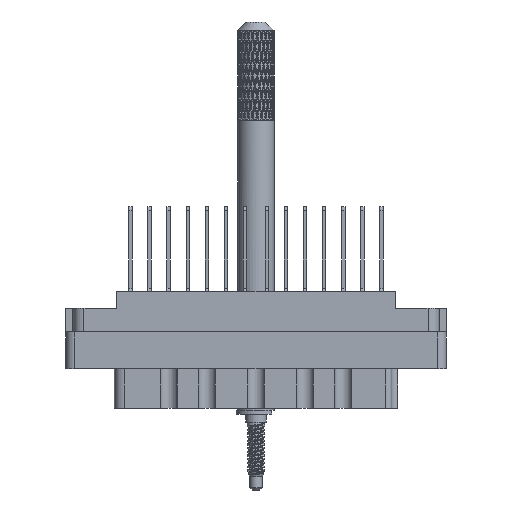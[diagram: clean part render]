
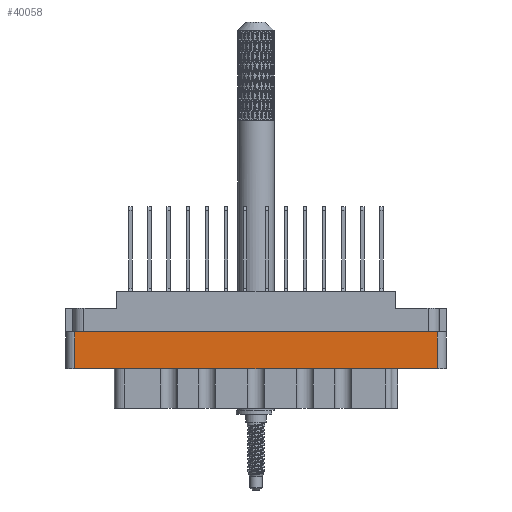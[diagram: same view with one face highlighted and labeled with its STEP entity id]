
A CAD part, front view. The second image highlights one B-rep face of the part: STEP entity #40058.
In plain terms, the highlighted planar face has unit normal (0, -1, 0).
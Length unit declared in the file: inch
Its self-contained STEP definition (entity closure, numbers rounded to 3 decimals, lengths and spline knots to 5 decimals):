
#10242 = DIRECTION ( 'NONE',  ( 0., -1., 0. ) ) ;
#10829 = FACE_OUTER_BOUND ( 'NONE', #108173, .T. ) ;
#15370 = ORIENTED_EDGE ( 'NONE', *, *, #99197, .F. ) ;
#15640 = CARTESIAN_POINT ( 'NONE',  ( 1.234, -0.438, -0.798 ) ) ;
#28020 = CARTESIAN_POINT ( 'NONE',  ( 0., -0.438, -0.529 ) ) ;
#29146 = CARTESIAN_POINT ( 'NONE',  ( -1.296, -0.438, -0.798 ) ) ;
#30642 = VERTEX_POINT ( 'NONE', #67618 ) ;
#34133 = DIRECTION ( 'NONE',  ( 0., 0., 1. ) ) ;
#37574 = VECTOR ( 'NONE', #46187, 39.37008 ) ;
#40058 = ADVANCED_FACE ( 'NONE', ( #10829 ), #91553, .T. ) ;
#45453 = ORIENTED_EDGE ( 'NONE', *, *, #83972, .F. ) ;
#46187 = DIRECTION ( 'NONE',  ( -1., 0., 0. ) ) ;
#47696 = DIRECTION ( 'NONE',  ( 0., 0., -1. ) ) ;
#49964 = AXIS2_PLACEMENT_3D ( 'NONE', #29146, #10242, #47696 ) ;
#51877 = CARTESIAN_POINT ( 'NONE',  ( 1.234, -0.438, -0.277 ) ) ;
#53522 = DIRECTION ( 'NONE',  ( 1., 0., 0. ) ) ;
#61423 = VERTEX_POINT ( 'NONE', #98308 ) ;
#61961 = DIRECTION ( 'NONE',  ( 0., 0., -1. ) ) ;
#67618 = CARTESIAN_POINT ( 'NONE',  ( -1.234, -0.438, -0.529 ) ) ;
#68690 = VERTEX_POINT ( 'NONE', #51877 ) ;
#70128 = CARTESIAN_POINT ( 'NONE',  ( 0., -0.438, -0.277 ) ) ;
#71043 = CARTESIAN_POINT ( 'NONE',  ( -1.234, -0.438, -0.798 ) ) ;
#77001 = VECTOR ( 'NONE', #53522, 39.37008 ) ;
#78864 = VECTOR ( 'NONE', #61961, 39.37008 ) ;
#79878 = LINE ( 'NONE', #70128, #77001 ) ;
#81186 = VERTEX_POINT ( 'NONE', #84804 ) ;
#81673 = LINE ( 'NONE', #71043, #78864 ) ;
#83972 = EDGE_CURVE ( 'NONE', #61423, #68690, #79878, .T. ) ;
#84804 = CARTESIAN_POINT ( 'NONE',  ( 1.234, -0.438, -0.529 ) ) ;
#87998 = VECTOR ( 'NONE', #34133, 39.37008 ) ;
#90091 = ORIENTED_EDGE ( 'NONE', *, *, #114015, .T. ) ;
#91553 = PLANE ( 'NONE',  #49964 ) ;
#91884 = ORIENTED_EDGE ( 'NONE', *, *, #108337, .T. ) ;
#98308 = CARTESIAN_POINT ( 'NONE',  ( -1.234, -0.438, -0.277 ) ) ;
#99197 = EDGE_CURVE ( 'NONE', #81186, #30642, #113706, .T. ) ;
#108173 = EDGE_LOOP ( 'NONE', ( #45453, #91884, #15370, #90091 ) ) ;
#108337 = EDGE_CURVE ( 'NONE', #61423, #30642, #81673, .T. ) ;
#111876 = LINE ( 'NONE', #15640, #87998 ) ;
#113706 = LINE ( 'NONE', #28020, #37574 ) ;
#114015 = EDGE_CURVE ( 'NONE', #81186, #68690, #111876, .T. ) ;
